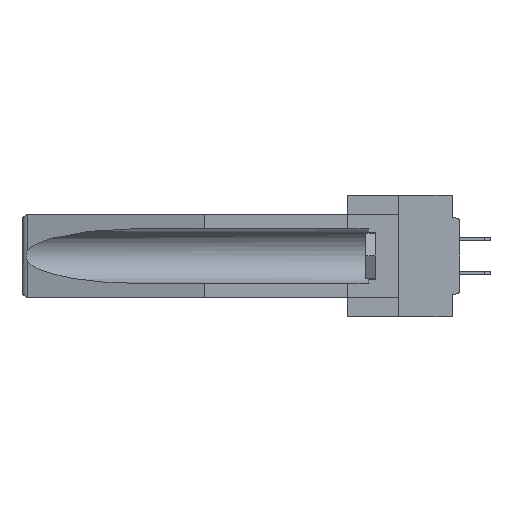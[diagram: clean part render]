
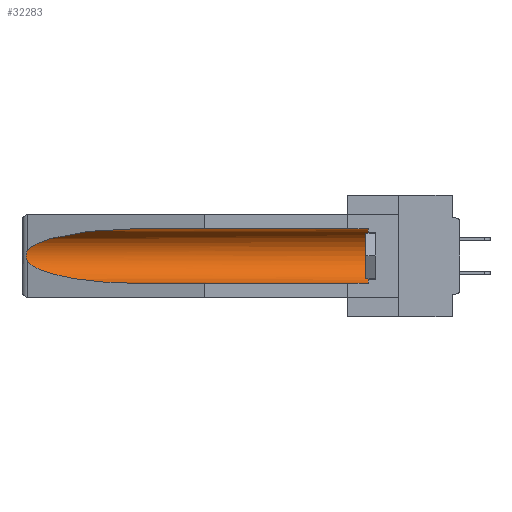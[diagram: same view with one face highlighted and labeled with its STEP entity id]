
A CAD part, left-side view. The second image highlights one B-rep face of the part: STEP entity #32283.
In plain terms, the highlighted cylindrical face has radius 2.857 mm (diameter 5.715 mm), a partial arc.
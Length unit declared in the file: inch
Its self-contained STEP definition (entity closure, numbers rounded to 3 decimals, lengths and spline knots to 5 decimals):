
#103 = CARTESIAN_POINT ( 'NONE',  ( 0.155, 0.126, -0.059 ) ) ;
#348 = LINE ( 'NONE', #12155, #35101 ) ;
#854 = DIRECTION ( 'NONE',  ( 0., -1., 0. ) ) ;
#878 = ORIENTED_EDGE ( 'NONE', *, *, #27394, .T. ) ;
#1301 = CARTESIAN_POINT ( 'NONE',  ( 0.26537, 1.52718, -0.19328 ) ) ;
#2013 = CARTESIAN_POINT ( 'NONE',  ( 0.155, 1.07973, -0.059 ) ) ;
#2674 = CARTESIAN_POINT ( 'NONE',  ( 0.26537, 1.52718, -0.14972 ) ) ;
#3671 = FACE_OUTER_BOUND ( 'NONE', #12954, .T. ) ;
#3715 = VERTEX_POINT ( 'NONE', #35063 ) ;
#4546 = DIRECTION ( 'NONE',  ( 0., 0., 1. ) ) ;
#4909 = CARTESIAN_POINT ( 'NONE',  ( 0.25451, 1.48313, -0.24835 ) ) ;
#5152 = CARTESIAN_POINT ( 'NONE',  ( 0.26537, 1.52718, -0.14972 ) ) ;
#6126 =( BOUNDED_CURVE ( )  B_SPLINE_CURVE ( 3, ( #28977, #4909, #35837, #32496 ),
 .UNSPECIFIED., .F., .F. ) 
 B_SPLINE_CURVE_WITH_KNOTS ( ( 4, 4 ),
 ( 0.1948, 1.5708 ),
 .UNSPECIFIED. ) 
 CURVE ( )  GEOMETRIC_REPRESENTATION_ITEM ( )  RATIONAL_B_SPLINE_CURVE ( ( 1., 0.848, 0.848, 1. ) ) 
 REPRESENTATION_ITEM ( '' )  );
#9149 = DIRECTION ( 'NONE',  ( 0., 0., 1. ) ) ;
#10420 = AXIS2_PLACEMENT_3D ( 'NONE', #15130, #854, #4546 ) ;
#12155 = CARTESIAN_POINT ( 'NONE',  ( 0.155, -0.30754, -0.059 ) ) ;
#12213 = EDGE_CURVE ( 'NONE', #21365, #14103, #6126, .T. ) ;
#12256 = CARTESIAN_POINT ( 'NONE',  ( 0.26597, 1.5296, -0.19026 ) ) ;
#12396 = CARTESIAN_POINT ( 'NONE',  ( 0.2675, 1.53308, -0.17534 ) ) ;
#12927 = CYLINDRICAL_SURFACE ( 'NONE', #26925, 0.1125 ) ;
#12954 = EDGE_LOOP ( 'NONE', ( #878, #27754, #24102, #26756, #27367, #33245 ) ) ;
#14103 = VERTEX_POINT ( 'NONE', #30427 ) ;
#14835 = VECTOR ( 'NONE', #31212, 39.37008 ) ;
#15130 = CARTESIAN_POINT ( 'NONE',  ( 0.155, 0.126, -0.1715 ) ) ;
#15569 = CARTESIAN_POINT ( 'NONE',  ( 0.26655, 1.53094, -0.18657 ) ) ;
#15928 = CARTESIAN_POINT ( 'NONE',  ( 0.155, -0.30754, -0.1715 ) ) ;
#18762 = CARTESIAN_POINT ( 'NONE',  ( 0.2673, 1.53269, -0.17917 ) ) ;
#21365 = VERTEX_POINT ( 'NONE', #43059 ) ;
#23996 = LINE ( 'NONE', #27860, #14835 ) ;
#24102 = ORIENTED_EDGE ( 'NONE', *, *, #12213, .T. ) ;
#24397 = VERTEX_POINT ( 'NONE', #2013 ) ;
#25597 = EDGE_CURVE ( 'NONE', #32262, #14103, #23996, .T. ) ;
#25732 = CARTESIAN_POINT ( 'NONE',  ( 0.26654, 1.53092, -0.15636 ) ) ;
#26089 = CARTESIAN_POINT ( 'NONE',  ( 0.155, 0.126, -0.284 ) ) ;
#26756 = ORIENTED_EDGE ( 'NONE', *, *, #25597, .F. ) ;
#26925 = AXIS2_PLACEMENT_3D ( 'NONE', #15928, #29884, #9149 ) ;
#27027 = VERTEX_POINT ( 'NONE', #103 ) ;
#27367 = ORIENTED_EDGE ( 'NONE', *, *, #39038, .T. ) ;
#27394 = EDGE_CURVE ( 'NONE', #24397, #3715, #27773, .T. ) ;
#27754 = ORIENTED_EDGE ( 'NONE', *, *, #44249, .T. ) ;
#27773 =( BOUNDED_CURVE ( )  B_SPLINE_CURVE ( 3, ( #40878, #37262, #44099, #2674 ),
 .UNSPECIFIED., .F., .F. ) 
 B_SPLINE_CURVE_WITH_KNOTS ( ( 4, 4 ),
 ( 4.71239, 6.08839 ),
 .UNSPECIFIED. ) 
 CURVE ( )  GEOMETRIC_REPRESENTATION_ITEM ( )  RATIONAL_B_SPLINE_CURVE ( ( 1., 0.848, 0.848, 1. ) ) 
 REPRESENTATION_ITEM ( '' )  );
#27860 = CARTESIAN_POINT ( 'NONE',  ( 0.155, -0.30754, -0.284 ) ) ;
#28977 = CARTESIAN_POINT ( 'NONE',  ( 0.26537, 1.52718, -0.19328 ) ) ;
#29212 = CARTESIAN_POINT ( 'NONE',  ( 0.26597, 1.52961, -0.15275 ) ) ;
#29884 = DIRECTION ( 'NONE',  ( 0., 1., 0. ) ) ;
#30427 = CARTESIAN_POINT ( 'NONE',  ( 0.155, 1.07973, -0.284 ) ) ;
#31212 = DIRECTION ( 'NONE',  ( 0., 1., 0. ) ) ;
#32262 = VERTEX_POINT ( 'NONE', #26089 ) ;
#32283 = ADVANCED_FACE ( 'NONE', ( #3671 ), #12927, .F. ) ;
#32496 = CARTESIAN_POINT ( 'NONE',  ( 0.155, 1.07973, -0.284 ) ) ;
#32906 = EDGE_CURVE ( 'NONE', #27027, #24397, #348, .T. ) ;
#33024 = CARTESIAN_POINT ( 'NONE',  ( 0.2673, 1.5327, -0.16383 ) ) ;
#33245 = ORIENTED_EDGE ( 'NONE', *, *, #32906, .T. ) ;
#35063 = CARTESIAN_POINT ( 'NONE',  ( 0.26537, 1.52718, -0.14972 ) ) ;
#35101 = VECTOR ( 'NONE', #43531, 39.37008 ) ;
#35472 = CIRCLE ( 'NONE', #10420, 0.1125 ) ;
#35837 = CARTESIAN_POINT ( 'NONE',  ( 0.21114, 1.30732, -0.284 ) ) ;
#36368 = CARTESIAN_POINT ( 'NONE',  ( 0.2675, 1.53308, -0.16763 ) ) ;
#37262 = CARTESIAN_POINT ( 'NONE',  ( 0.21114, 1.30732, -0.059 ) ) ;
#39038 = EDGE_CURVE ( 'NONE', #32262, #27027, #35472, .T. ) ;
#40878 = CARTESIAN_POINT ( 'NONE',  ( 0.155, 1.07973, -0.059 ) ) ;
#41354 = B_SPLINE_CURVE_WITH_KNOTS ( 'NONE', 3,
 ( #5152, #29212, #25732, #33024, #36368, #12396, #18762, #15569, #12256, #1301 ),
 .UNSPECIFIED., .F., .F.,
 ( 4, 2, 2, 2, 4 ),
 ( 0., 0.00029, 0.00058, 0.00087, 0.00117 ),
 .UNSPECIFIED. ) ;
#43059 = CARTESIAN_POINT ( 'NONE',  ( 0.26537, 1.52718, -0.19328 ) ) ;
#43531 = DIRECTION ( 'NONE',  ( 0., 1., 0. ) ) ;
#44099 = CARTESIAN_POINT ( 'NONE',  ( 0.25451, 1.48313, -0.09465 ) ) ;
#44249 = EDGE_CURVE ( 'NONE', #3715, #21365, #41354, .T. ) ;
